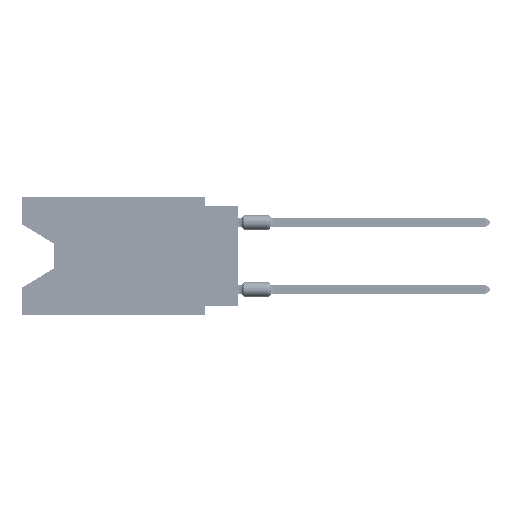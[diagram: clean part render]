
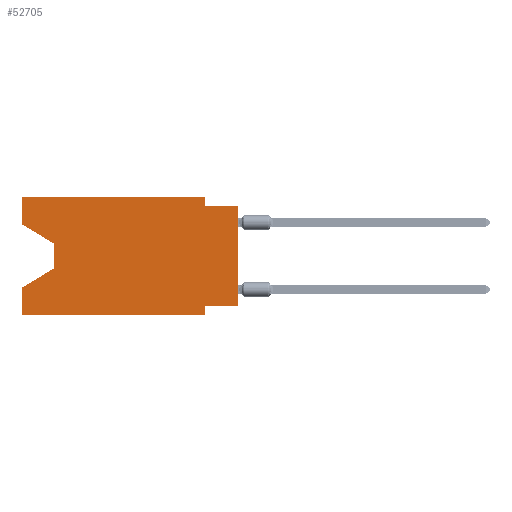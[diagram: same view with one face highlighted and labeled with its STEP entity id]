
A CAD part, left-side view. The second image highlights one B-rep face of the part: STEP entity #52705.
In plain terms, the highlighted planar face has unit normal (-1, 0, 0).
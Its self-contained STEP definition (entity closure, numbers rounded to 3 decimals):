
#32 = EDGE_CURVE ( 'NONE', #109097, #4992, #81382, .T. ) ;
#307 = EDGE_LOOP ( 'NONE', ( #79755, #106812, #54692, #98057, #59899, #25482, #95526, #56395, #22152, #7740, #15821, #67689 ) ) ;
#414 = CARTESIAN_POINT ( 'NONE',  ( 0., 0., -8.255 ) ) ;
#2153 = LINE ( 'NONE', #107741, #52067 ) ;
#3160 = DIRECTION ( 'NONE',  ( 0., -0.855, -0.519 ) ) ;
#3833 = LINE ( 'NONE', #100769, #94486 ) ;
#4685 = VERTEX_POINT ( 'NONE', #6620 ) ;
#4772 = AXIS2_PLACEMENT_3D ( 'NONE', #31924, #86129, #50948 ) ;
#4992 = VERTEX_POINT ( 'NONE', #72883 ) ;
#5976 = VERTEX_POINT ( 'NONE', #23390 ) ;
#6153 = VECTOR ( 'NONE', #102690, 1000. ) ;
#6620 = CARTESIAN_POINT ( 'NONE',  ( 0., 16.383, -8.89 ) ) ;
#7740 = ORIENTED_EDGE ( 'NONE', *, *, #32, .F. ) ;
#10343 = EDGE_CURVE ( 'NONE', #56161, #27693, #60187, .T. ) ;
#11559 = DIRECTION ( 'NONE',  ( 0., 0., -1. ) ) ;
#12276 = CARTESIAN_POINT ( 'NONE',  ( 0., 2.54, -8.89 ) ) ;
#13676 = VERTEX_POINT ( 'NONE', #12276 ) ;
#13799 = VECTOR ( 'NONE', #3160, 1000. ) ;
#15821 = ORIENTED_EDGE ( 'NONE', *, *, #40754, .F. ) ;
#20400 = EDGE_CURVE ( 'NONE', #56161, #5976, #110459, .T. ) ;
#20966 = VERTEX_POINT ( 'NONE', #43358 ) ;
#21038 = CARTESIAN_POINT ( 'NONE',  ( 0., 16.383, -2.038 ) ) ;
#22032 = VERTEX_POINT ( 'NONE', #63643 ) ;
#22142 = LINE ( 'NONE', #57320, #81624 ) ;
#22152 = ORIENTED_EDGE ( 'NONE', *, *, #42711, .F. ) ;
#23390 = CARTESIAN_POINT ( 'NONE',  ( 0., 13.97, -3.505 ) ) ;
#24897 = VECTOR ( 'NONE', #69965, 1000. ) ;
#25139 = CARTESIAN_POINT ( 'NONE',  ( 0., 13.97, -5.385 ) ) ;
#25482 = ORIENTED_EDGE ( 'NONE', *, *, #65500, .F. ) ;
#25658 = EDGE_CURVE ( 'NONE', #4685, #101509, #2153, .T. ) ;
#27693 = VERTEX_POINT ( 'NONE', #93423 ) ;
#31130 = LINE ( 'NONE', #82475, #67206 ) ;
#31697 = LINE ( 'NONE', #68005, #68110 ) ;
#31924 = CARTESIAN_POINT ( 'NONE',  ( 0., 16.383, 0. ) ) ;
#31958 = DIRECTION ( 'NONE',  ( 0., 0., 1. ) ) ;
#38124 = CARTESIAN_POINT ( 'NONE',  ( 0., 2.54, 0. ) ) ;
#38441 = CARTESIAN_POINT ( 'NONE',  ( 0., 16.383, -2.038 ) ) ;
#40754 = EDGE_CURVE ( 'NONE', #27693, #109097, #22142, .T. ) ;
#41891 = VERTEX_POINT ( 'NONE', #102338 ) ;
#42000 = LINE ( 'NONE', #77188, #61076 ) ;
#42313 = CARTESIAN_POINT ( 'NONE',  ( 0., 16.383, 0. ) ) ;
#42711 = EDGE_CURVE ( 'NONE', #4992, #22032, #31130, .T. ) ;
#43358 = CARTESIAN_POINT ( 'NONE',  ( 0., 0., -8.255 ) ) ;
#50948 = DIRECTION ( 'NONE',  ( 0., 0., -1. ) ) ;
#52067 = VECTOR ( 'NONE', #31958, 1000. ) ;
#52705 = ADVANCED_FACE ( 'NONE', ( #101728 ), #59586, .F. ) ;
#54555 = VECTOR ( 'NONE', #63275, 1000. ) ;
#54692 = ORIENTED_EDGE ( 'NONE', *, *, #112383, .T. ) ;
#56161 = VERTEX_POINT ( 'NONE', #38441 ) ;
#56395 = ORIENTED_EDGE ( 'NONE', *, *, #104291, .T. ) ;
#56913 = DIRECTION ( 'NONE',  ( 0., -1., 0. ) ) ;
#57320 = CARTESIAN_POINT ( 'NONE',  ( 0., 16.383, 0. ) ) ;
#58046 = DIRECTION ( 'NONE',  ( 0., 0., -1. ) ) ;
#58834 = LINE ( 'NONE', #59980, #6153 ) ;
#59586 = PLANE ( 'NONE',  #4772 ) ;
#59899 = ORIENTED_EDGE ( 'NONE', *, *, #66887, .T. ) ;
#59980 = CARTESIAN_POINT ( 'NONE',  ( 0., 0., 0. ) ) ;
#60187 = LINE ( 'NONE', #42313, #24897 ) ;
#61076 = VECTOR ( 'NONE', #86396, 1000. ) ;
#62522 = EDGE_CURVE ( 'NONE', #5976, #93587, #84023, .T. ) ;
#63275 = DIRECTION ( 'NONE',  ( 0., 1., 0. ) ) ;
#63643 = CARTESIAN_POINT ( 'NONE',  ( 0., 0., -0.635 ) ) ;
#65500 = EDGE_CURVE ( 'NONE', #41891, #13676, #42000, .T. ) ;
#66233 = CARTESIAN_POINT ( 'NONE',  ( 0., 16.383, -6.852 ) ) ;
#66887 = EDGE_CURVE ( 'NONE', #4685, #13676, #3833, .T. ) ;
#67206 = VECTOR ( 'NONE', #83033, 1000. ) ;
#67689 = ORIENTED_EDGE ( 'NONE', *, *, #10343, .F. ) ;
#68005 = CARTESIAN_POINT ( 'NONE',  ( 0., 13.97, -5.385 ) ) ;
#68110 = VECTOR ( 'NONE', #103214, 1000. ) ;
#69965 = DIRECTION ( 'NONE',  ( 0., 0., 1. ) ) ;
#72883 = CARTESIAN_POINT ( 'NONE',  ( 0., 2.54, -0.635 ) ) ;
#76132 = VECTOR ( 'NONE', #58046, 1000. ) ;
#77188 = CARTESIAN_POINT ( 'NONE',  ( 0., 2.54, -8.89 ) ) ;
#79755 = ORIENTED_EDGE ( 'NONE', *, *, #20400, .T. ) ;
#80015 = LINE ( 'NONE', #414, #54555 ) ;
#81382 = LINE ( 'NONE', #38124, #102917 ) ;
#81624 = VECTOR ( 'NONE', #92493, 1000. ) ;
#82475 = CARTESIAN_POINT ( 'NONE',  ( 0., 0., -0.635 ) ) ;
#83033 = DIRECTION ( 'NONE',  ( 0., -1., 0. ) ) ;
#84023 = LINE ( 'NONE', #110012, #76132 ) ;
#84543 = CARTESIAN_POINT ( 'NONE',  ( 0., 2.54, 0. ) ) ;
#86129 = DIRECTION ( 'NONE',  ( 1., 0., 0. ) ) ;
#86396 = DIRECTION ( 'NONE',  ( 0., 0., -1. ) ) ;
#88881 = EDGE_CURVE ( 'NONE', #20966, #41891, #80015, .T. ) ;
#92493 = DIRECTION ( 'NONE',  ( 0., -1., 0. ) ) ;
#93423 = CARTESIAN_POINT ( 'NONE',  ( 0., 16.383, 0. ) ) ;
#93587 = VERTEX_POINT ( 'NONE', #25139 ) ;
#94486 = VECTOR ( 'NONE', #56913, 1000. ) ;
#95526 = ORIENTED_EDGE ( 'NONE', *, *, #88881, .F. ) ;
#98057 = ORIENTED_EDGE ( 'NONE', *, *, #25658, .F. ) ;
#100769 = CARTESIAN_POINT ( 'NONE',  ( 0., 16.383, -8.89 ) ) ;
#101509 = VERTEX_POINT ( 'NONE', #66233 ) ;
#101728 = FACE_OUTER_BOUND ( 'NONE', #307, .T. ) ;
#102338 = CARTESIAN_POINT ( 'NONE',  ( 0., 2.54, -8.255 ) ) ;
#102690 = DIRECTION ( 'NONE',  ( 0., 0., 1. ) ) ;
#102917 = VECTOR ( 'NONE', #11559, 1000. ) ;
#103214 = DIRECTION ( 'NONE',  ( 0., 0.855, -0.519 ) ) ;
#104291 = EDGE_CURVE ( 'NONE', #20966, #22032, #58834, .T. ) ;
#106812 = ORIENTED_EDGE ( 'NONE', *, *, #62522, .T. ) ;
#107741 = CARTESIAN_POINT ( 'NONE',  ( 0., 16.383, 0. ) ) ;
#109097 = VERTEX_POINT ( 'NONE', #84543 ) ;
#110012 = CARTESIAN_POINT ( 'NONE',  ( 0., 13.97, -3.505 ) ) ;
#110459 = LINE ( 'NONE', #21038, #13799 ) ;
#112383 = EDGE_CURVE ( 'NONE', #93587, #101509, #31697, .T. ) ;
